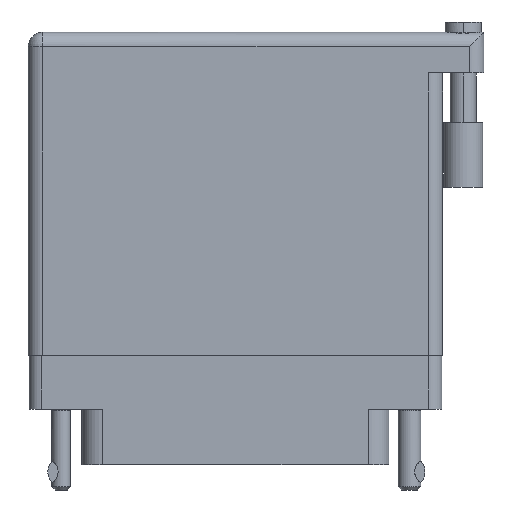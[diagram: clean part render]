
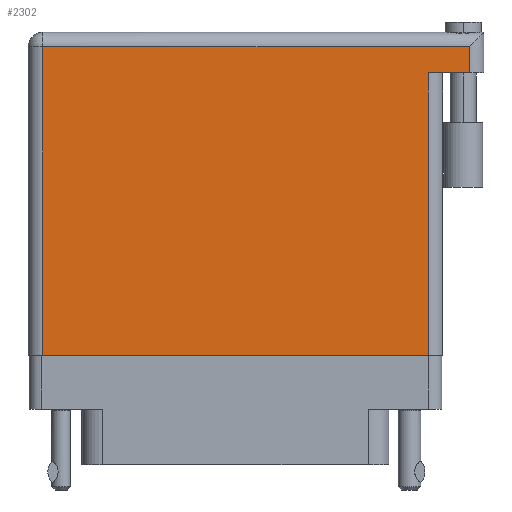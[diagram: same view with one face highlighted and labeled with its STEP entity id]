
A CAD part, front view. The second image highlights one B-rep face of the part: STEP entity #2302.
In plain terms, the highlighted face is planar.
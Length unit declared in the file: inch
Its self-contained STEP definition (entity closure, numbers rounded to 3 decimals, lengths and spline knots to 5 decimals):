
#841 = EDGE_CURVE ( 'NONE', #31737, #3275, #24748, .T. ) ;
#2235 = EDGE_CURVE ( 'NONE', #45600, #20150, #7110, .T. ) ;
#2302 = ADVANCED_FACE ( 'NONE', ( #4678 ), #4427, .F. ) ;
#3275 = VERTEX_POINT ( 'NONE', #45226 ) ;
#3924 = CARTESIAN_POINT ( 'NONE',  ( 2.138, 1.496, 0. ) ) ;
#4427 = PLANE ( 'NONE',  #34588 ) ;
#4678 = FACE_OUTER_BOUND ( 'NONE', #10906, .T. ) ;
#6584 = CARTESIAN_POINT ( 'NONE',  ( 0., 0., 0. ) ) ;
#7110 = LINE ( 'NONE', #36653, #47733 ) ;
#8067 = DIRECTION ( 'NONE',  ( -1., 0., 0. ) ) ;
#10634 = LINE ( 'NONE', #36550, #22687 ) ;
#10806 = CARTESIAN_POINT ( 'NONE',  ( 0.07, 1.496, 0. ) ) ;
#10906 = EDGE_LOOP ( 'NONE', ( #35271, #20903, #14016, #18246, #24625, #22256 ) ) ;
#14016 = ORIENTED_EDGE ( 'NONE', *, *, #2235, .F. ) ;
#14773 = CARTESIAN_POINT ( 'NONE',  ( 0.07, 0., 0. ) ) ;
#16542 = VECTOR ( 'NONE', #46732, 39.37008 ) ;
#16868 = EDGE_CURVE ( 'NONE', #25139, #35347, #43935, .T. ) ;
#16953 = VECTOR ( 'NONE', #44183, 39.37008 ) ;
#18246 = ORIENTED_EDGE ( 'NONE', *, *, #44668, .T. ) ;
#19209 = DIRECTION ( 'NONE',  ( 0., 0., -1. ) ) ;
#20150 = VERTEX_POINT ( 'NONE', #39819 ) ;
#20903 = ORIENTED_EDGE ( 'NONE', *, *, #45323, .T. ) ;
#21550 = DIRECTION ( 'NONE',  ( 0., -1., 0. ) ) ;
#22256 = ORIENTED_EDGE ( 'NONE', *, *, #33884, .T. ) ;
#22687 = VECTOR ( 'NONE', #25400, 39.37008 ) ;
#24625 = ORIENTED_EDGE ( 'NONE', *, *, #16868, .T. ) ;
#24748 = LINE ( 'NONE', #6584, #26272 ) ;
#25139 = VERTEX_POINT ( 'NONE', #3924 ) ;
#25400 = DIRECTION ( 'NONE',  ( 0., 1., 0. ) ) ;
#26272 = VECTOR ( 'NONE', #35652, 39.37008 ) ;
#26478 = VECTOR ( 'NONE', #21550, 39.37008 ) ;
#30205 = CARTESIAN_POINT ( 'NONE',  ( 1.938, 1.369, 0. ) ) ;
#31717 = CARTESIAN_POINT ( 'NONE',  ( 0., 1.566, 0. ) ) ;
#31737 = VERTEX_POINT ( 'NONE', #34153 ) ;
#33884 = EDGE_CURVE ( 'NONE', #35347, #31737, #39972, .T. ) ;
#34153 = CARTESIAN_POINT ( 'NONE',  ( 0.07, 0., 0. ) ) ;
#34588 = AXIS2_PLACEMENT_3D ( 'NONE', #31717, #19209, #8067 ) ;
#35271 = ORIENTED_EDGE ( 'NONE', *, *, #841, .T. ) ;
#35347 = VERTEX_POINT ( 'NONE', #10806 ) ;
#35652 = DIRECTION ( 'NONE',  ( 1., 0., 0. ) ) ;
#36550 = CARTESIAN_POINT ( 'NONE',  ( 2.138, 1.566, 0. ) ) ;
#36653 = CARTESIAN_POINT ( 'NONE',  ( 2.208, 1.369, 0. ) ) ;
#38161 = CARTESIAN_POINT ( 'NONE',  ( 2.138, 1.369, 0. ) ) ;
#39819 = CARTESIAN_POINT ( 'NONE',  ( 1.938, 1.369, 0. ) ) ;
#39972 = LINE ( 'NONE', #14773, #26478 ) ;
#40541 = DIRECTION ( 'NONE',  ( -1., 0., 0. ) ) ;
#43237 = CARTESIAN_POINT ( 'NONE',  ( 0., 1.496, 0. ) ) ;
#43935 = LINE ( 'NONE', #43237, #16953 ) ;
#44183 = DIRECTION ( 'NONE',  ( -1., 0., 0. ) ) ;
#44532 = LINE ( 'NONE', #30205, #16542 ) ;
#44668 = EDGE_CURVE ( 'NONE', #45600, #25139, #10634, .T. ) ;
#45226 = CARTESIAN_POINT ( 'NONE',  ( 1.938, 0., 0. ) ) ;
#45323 = EDGE_CURVE ( 'NONE', #3275, #20150, #44532, .T. ) ;
#45600 = VERTEX_POINT ( 'NONE', #38161 ) ;
#46732 = DIRECTION ( 'NONE',  ( 0., 1., 0. ) ) ;
#47733 = VECTOR ( 'NONE', #40541, 39.37008 ) ;
